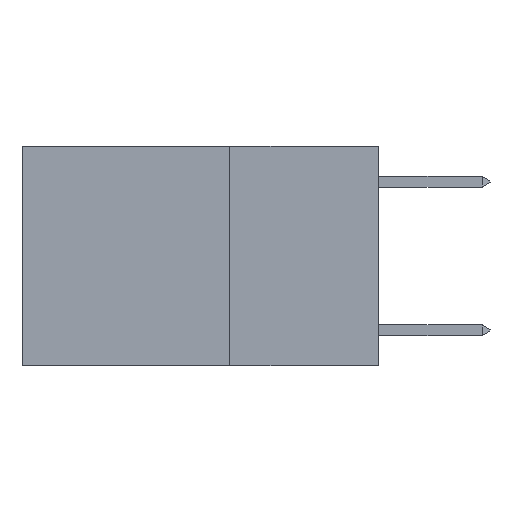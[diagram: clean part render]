
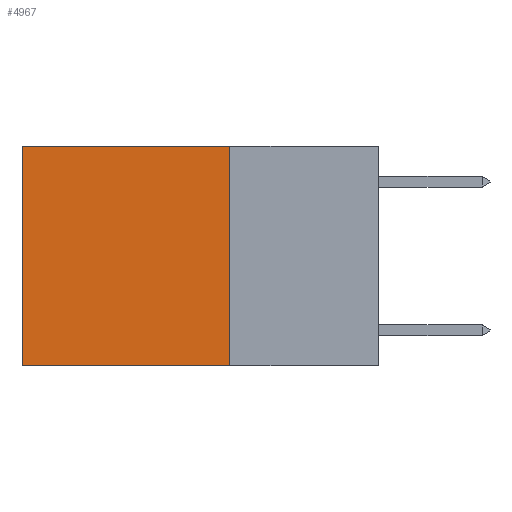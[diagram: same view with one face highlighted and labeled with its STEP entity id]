
A CAD part, left-side view. The second image highlights one B-rep face of the part: STEP entity #4967.
In plain terms, the highlighted planar face has unit normal (-1, 0, 0).
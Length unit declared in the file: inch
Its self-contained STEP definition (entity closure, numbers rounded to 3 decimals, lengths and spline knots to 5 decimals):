
#2218 = ORIENTED_EDGE ( 'NONE', *, *, #11528, .F. ) ;
#2335 = CARTESIAN_POINT ( 'NONE',  ( 0.2625, 0.6, -0.37 ) ) ;
#2716 = AXIS2_PLACEMENT_3D ( 'NONE', #17545, #6580, #3551 ) ;
#3369 = ORIENTED_EDGE ( 'NONE', *, *, #8271, .T. ) ;
#3551 = DIRECTION ( 'NONE',  ( 0., 0., -1. ) ) ;
#3772 = CARTESIAN_POINT ( 'NONE',  ( 0.2625, 0.25, -0.37 ) ) ;
#3821 = EDGE_LOOP ( 'NONE', ( #3369, #13066, #2218, #14386 ) ) ;
#3892 = CARTESIAN_POINT ( 'NONE',  ( 0.2625, 0.25, 0. ) ) ;
#3944 = LINE ( 'NONE', #11583, #8244 ) ;
#4967 = ADVANCED_FACE ( 'NONE', ( #5368 ), #11123, .F. ) ;
#5368 = FACE_OUTER_BOUND ( 'NONE', #3821, .T. ) ;
#5693 = VECTOR ( 'NONE', #16611, 39.37008 ) ;
#6580 = DIRECTION ( 'NONE',  ( 1., 0., 0. ) ) ;
#8244 = VECTOR ( 'NONE', #8365, 39.37008 ) ;
#8271 = EDGE_CURVE ( 'NONE', #14780, #19123, #12284, .T. ) ;
#8365 = DIRECTION ( 'NONE',  ( 0., 0., -1. ) ) ;
#9372 = CARTESIAN_POINT ( 'NONE',  ( 0.2625, 0.6, 0. ) ) ;
#9719 = VERTEX_POINT ( 'NONE', #3772 ) ;
#10284 = CARTESIAN_POINT ( 'NONE',  ( 0.2625, 0.25, -0.37 ) ) ;
#11123 = PLANE ( 'NONE',  #2716 ) ;
#11473 = VECTOR ( 'NONE', #15199, 39.37008 ) ;
#11528 = EDGE_CURVE ( 'NONE', #17323, #9719, #3944, .T. ) ;
#11583 = CARTESIAN_POINT ( 'NONE',  ( 0.2625, 0.25, 0. ) ) ;
#11682 = EDGE_CURVE ( 'NONE', #9719, #19123, #13501, .T. ) ;
#12284 = LINE ( 'NONE', #9372, #11473 ) ;
#13066 = ORIENTED_EDGE ( 'NONE', *, *, #11682, .F. ) ;
#13501 = LINE ( 'NONE', #10284, #5693 ) ;
#14386 = ORIENTED_EDGE ( 'NONE', *, *, #17979, .T. ) ;
#14780 = VERTEX_POINT ( 'NONE', #15610 ) ;
#14815 = LINE ( 'NONE', #18167, #16134 ) ;
#15199 = DIRECTION ( 'NONE',  ( 0., 0., -1. ) ) ;
#15610 = CARTESIAN_POINT ( 'NONE',  ( 0.2625, 0.6, 0. ) ) ;
#16134 = VECTOR ( 'NONE', #16336, 39.37008 ) ;
#16336 = DIRECTION ( 'NONE',  ( 0., 1., 0. ) ) ;
#16611 = DIRECTION ( 'NONE',  ( 0., 1., 0. ) ) ;
#17323 = VERTEX_POINT ( 'NONE', #3892 ) ;
#17545 = CARTESIAN_POINT ( 'NONE',  ( 0.2625, 0.25, 0. ) ) ;
#17979 = EDGE_CURVE ( 'NONE', #17323, #14780, #14815, .T. ) ;
#18167 = CARTESIAN_POINT ( 'NONE',  ( 0.2625, 0.25, 0. ) ) ;
#19123 = VERTEX_POINT ( 'NONE', #2335 ) ;
